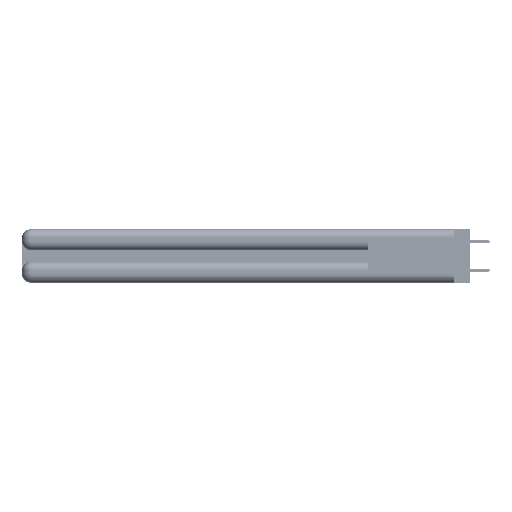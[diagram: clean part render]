
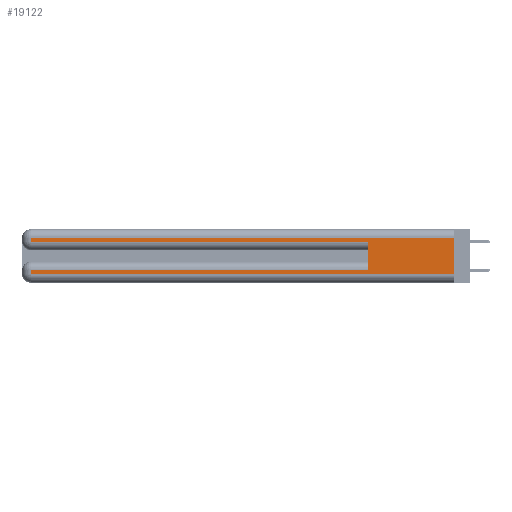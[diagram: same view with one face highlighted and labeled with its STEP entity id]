
A CAD part, left-side view. The second image highlights one B-rep face of the part: STEP entity #19122.
In plain terms, the highlighted planar face has unit normal (-1, 0, 0).
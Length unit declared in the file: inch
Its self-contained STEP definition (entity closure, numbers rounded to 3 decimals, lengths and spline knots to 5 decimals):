
#763 = LINE ( 'NONE', #39604, #46870 ) ;
#865 = CARTESIAN_POINT ( 'NONE',  ( 0., 0., 0.085 ) ) ;
#1285 = EDGE_CURVE ( 'NONE', #25827, #10573, #763, .T. ) ;
#1366 = VECTOR ( 'NONE', #33893, 39.37008 ) ;
#2308 = CARTESIAN_POINT ( 'NONE',  ( 0., 2.94, 0.37 ) ) ;
#3703 = CARTESIAN_POINT ( 'NONE',  ( 0., 0., 0.37 ) ) ;
#6133 = ORIENTED_EDGE ( 'NONE', *, *, #1285, .T. ) ;
#6916 = FACE_OUTER_BOUND ( 'NONE', #29303, .T. ) ;
#7247 = CARTESIAN_POINT ( 'NONE',  ( 0., 2.94, 0.37 ) ) ;
#8209 = DIRECTION ( 'NONE',  ( 0., 0., -1. ) ) ;
#9843 = LINE ( 'NONE', #865, #32231 ) ;
#10283 = DIRECTION ( 'NONE',  ( 0., 1., 0. ) ) ;
#10573 = VERTEX_POINT ( 'NONE', #47655 ) ;
#11317 = DIRECTION ( 'NONE',  ( 0., 0., -1. ) ) ;
#13260 = CARTESIAN_POINT ( 'NONE',  ( 0., 0.6, 0.085 ) ) ;
#14078 = VERTEX_POINT ( 'NONE', #25259 ) ;
#14381 = VERTEX_POINT ( 'NONE', #22684 ) ;
#14826 = VECTOR ( 'NONE', #8209, 39.37008 ) ;
#14948 = CARTESIAN_POINT ( 'NONE',  ( 0., 0., 0.06 ) ) ;
#16231 = LINE ( 'NONE', #3703, #14826 ) ;
#16448 = DIRECTION ( 'NONE',  ( 0., 0., -1. ) ) ;
#17502 = CARTESIAN_POINT ( 'NONE',  ( 0., 2.94, 0.085 ) ) ;
#18375 = CARTESIAN_POINT ( 'NONE',  ( 0., 0., 0.37 ) ) ;
#18686 = EDGE_CURVE ( 'NONE', #34883, #10573, #25181, .T. ) ;
#19122 = ADVANCED_FACE ( 'NONE', ( #6916 ), #45090, .F. ) ;
#19695 = VECTOR ( 'NONE', #45953, 39.37008 ) ;
#21762 = EDGE_CURVE ( 'NONE', #27337, #14078, #54901, .T. ) ;
#22684 = CARTESIAN_POINT ( 'NONE',  ( 0., 0., 0.06 ) ) ;
#22887 = DIRECTION ( 'NONE',  ( 0., 0., -1. ) ) ;
#25181 = LINE ( 'NONE', #47075, #1366 ) ;
#25259 = CARTESIAN_POINT ( 'NONE',  ( 0., 2.94, 0.06 ) ) ;
#25827 = VERTEX_POINT ( 'NONE', #43890 ) ;
#26006 = ORIENTED_EDGE ( 'NONE', *, *, #49523, .F. ) ;
#26163 = EDGE_CURVE ( 'NONE', #52672, #38664, #50290, .T. ) ;
#27337 = VERTEX_POINT ( 'NONE', #17502 ) ;
#29303 = EDGE_LOOP ( 'NONE', ( #26006, #34200, #54037, #6133, #52338, #48439, #34417, #36431 ) ) ;
#32174 = DIRECTION ( 'NONE',  ( 0., 1., 0. ) ) ;
#32231 = VECTOR ( 'NONE', #32174, 39.37008 ) ;
#33019 = LINE ( 'NONE', #14948, #19695 ) ;
#33893 = DIRECTION ( 'NONE',  ( 0., 0., 1. ) ) ;
#34200 = ORIENTED_EDGE ( 'NONE', *, *, #26163, .T. ) ;
#34417 = ORIENTED_EDGE ( 'NONE', *, *, #21762, .T. ) ;
#34883 = VERTEX_POINT ( 'NONE', #13260 ) ;
#36431 = ORIENTED_EDGE ( 'NONE', *, *, #56240, .T. ) ;
#38664 = VERTEX_POINT ( 'NONE', #51057 ) ;
#39604 = CARTESIAN_POINT ( 'NONE',  ( 0., 0., 0.285 ) ) ;
#40257 = DIRECTION ( 'NONE',  ( 0., -1., 0. ) ) ;
#42715 = EDGE_CURVE ( 'NONE', #38664, #25827, #56759, .T. ) ;
#43075 = VECTOR ( 'NONE', #11317, 39.37008 ) ;
#43438 = CARTESIAN_POINT ( 'NONE',  ( 0., 0., 0.31 ) ) ;
#43890 = CARTESIAN_POINT ( 'NONE',  ( 0., 2.94, 0.285 ) ) ;
#44910 = VECTOR ( 'NONE', #16448, 39.37008 ) ;
#45090 = PLANE ( 'NONE',  #50510 ) ;
#45953 = DIRECTION ( 'NONE',  ( 0., -1., 0. ) ) ;
#46870 = VECTOR ( 'NONE', #40257, 39.37008 ) ;
#47075 = CARTESIAN_POINT ( 'NONE',  ( 0., 0.6, 0.145 ) ) ;
#47655 = CARTESIAN_POINT ( 'NONE',  ( 0., 0.6, 0.285 ) ) ;
#48439 = ORIENTED_EDGE ( 'NONE', *, *, #50344, .T. ) ;
#49523 = EDGE_CURVE ( 'NONE', #52672, #14381, #16231, .T. ) ;
#49567 = DIRECTION ( 'NONE',  ( 1., 0., 0. ) ) ;
#50290 = LINE ( 'NONE', #54739, #54464 ) ;
#50344 = EDGE_CURVE ( 'NONE', #34883, #27337, #9843, .T. ) ;
#50510 = AXIS2_PLACEMENT_3D ( 'NONE', #18375, #49567, #22887 ) ;
#51057 = CARTESIAN_POINT ( 'NONE',  ( 0., 2.94, 0.31 ) ) ;
#52338 = ORIENTED_EDGE ( 'NONE', *, *, #18686, .F. ) ;
#52672 = VERTEX_POINT ( 'NONE', #43438 ) ;
#54037 = ORIENTED_EDGE ( 'NONE', *, *, #42715, .T. ) ;
#54464 = VECTOR ( 'NONE', #10283, 39.37008 ) ;
#54739 = CARTESIAN_POINT ( 'NONE',  ( 0., 0., 0.31 ) ) ;
#54901 = LINE ( 'NONE', #2308, #43075 ) ;
#56240 = EDGE_CURVE ( 'NONE', #14078, #14381, #33019, .T. ) ;
#56759 = LINE ( 'NONE', #7247, #44910 ) ;
